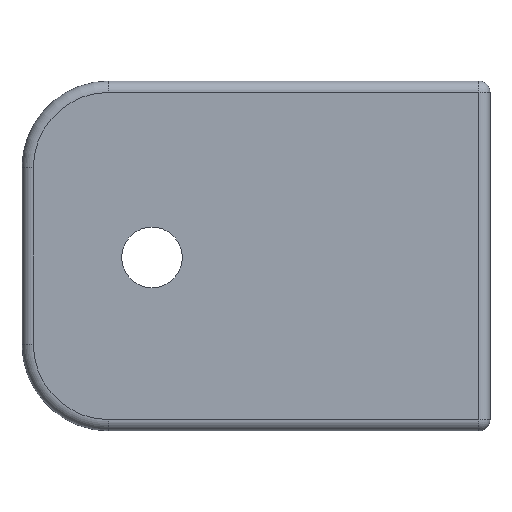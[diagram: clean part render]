
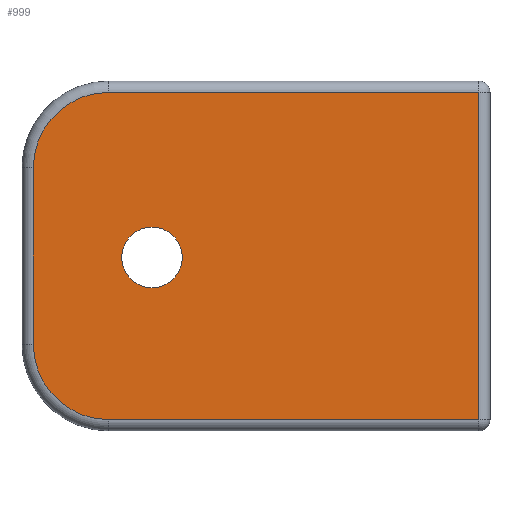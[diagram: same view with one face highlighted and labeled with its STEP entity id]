
A CAD part, front view. The second image highlights one B-rep face of the part: STEP entity #999.
In plain terms, the highlighted planar face has unit normal (0, -1, 0).
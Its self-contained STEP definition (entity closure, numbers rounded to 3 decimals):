
#17=FACE_BOUND('',#346,.T.);
#29=PLANE('',#1100);
#57=LINE('',#1514,#152);
#85=LINE('',#1604,#180);
#86=LINE('',#1608,#181);
#87=LINE('',#1612,#182);
#152=VECTOR('',#1199,10.);
#180=VECTOR('',#1291,10.);
#181=VECTOR('',#1296,10.);
#182=VECTOR('',#1299,10.);
#286=FACE_OUTER_BOUND('',#345,.T.);
#345=EDGE_LOOP('',(#765,#766,#767,#768,#769,#770));
#346=EDGE_LOOP('',(#771));
#413=CIRCLE('',#1101,6.62);
#414=CIRCLE('',#1102,6.62);
#415=CIRCLE('',#1103,2.667);
#442=VERTEX_POINT('',#1511);
#443=VERTEX_POINT('',#1513);
#473=VERTEX_POINT('',#1603);
#474=VERTEX_POINT('',#1607);
#475=VERTEX_POINT('',#1609);
#476=VERTEX_POINT('',#1611);
#477=VERTEX_POINT('',#1614);
#538=EDGE_CURVE('',#442,#443,#57,.T.);
#583=EDGE_CURVE('',#443,#473,#85,.T.);
#585=EDGE_CURVE('',#474,#442,#86,.T.);
#586=EDGE_CURVE('',#475,#474,#413,.T.);
#587=EDGE_CURVE('',#476,#475,#87,.T.);
#588=EDGE_CURVE('',#473,#476,#414,.T.);
#589=EDGE_CURVE('',#477,#477,#415,.T.);
#765=ORIENTED_EDGE('',*,*,#538,.F.);
#766=ORIENTED_EDGE('',*,*,#585,.F.);
#767=ORIENTED_EDGE('',*,*,#586,.F.);
#768=ORIENTED_EDGE('',*,*,#587,.F.);
#769=ORIENTED_EDGE('',*,*,#588,.F.);
#770=ORIENTED_EDGE('',*,*,#583,.F.);
#771=ORIENTED_EDGE('',*,*,#589,.T.);
#999=ADVANCED_FACE('',(#286,#17),#29,.F.);
#1100=AXIS2_PLACEMENT_3D('',#1606,#1294,#1295);
#1101=AXIS2_PLACEMENT_3D('',#1610,#1297,#1298);
#1102=AXIS2_PLACEMENT_3D('',#1613,#1300,#1301);
#1103=AXIS2_PLACEMENT_3D('',#1615,#1302,#1303);
#1199=DIRECTION('',(0.,0.,-1.));
#1291=DIRECTION('',(-1.,0.,0.));
#1294=DIRECTION('center_axis',(0.,1.,0.));
#1295=DIRECTION('ref_axis',(0.,0.,1.));
#1296=DIRECTION('',(1.,0.,0.));
#1297=DIRECTION('center_axis',(0.,1.,0.));
#1298=DIRECTION('ref_axis',(-0.707,0.,0.707));
#1299=DIRECTION('',(0.,0.,1.));
#1300=DIRECTION('center_axis',(0.,1.,0.));
#1301=DIRECTION('ref_axis',(-0.707,0.,-0.707));
#1302=DIRECTION('center_axis',(0.,1.,0.));
#1303=DIRECTION('ref_axis',(-1.,0.,0.));
#1511=CARTESIAN_POINT('',(40.01,-0.25,0.));
#1513=CARTESIAN_POINT('',(40.01,-0.25,-28.778));
#1514=CARTESIAN_POINT('',(40.01,-0.25,-7.195));
#1603=CARTESIAN_POINT('',(7.46,-0.25,-28.778));
#1604=CARTESIAN_POINT('',(29.489,-0.25,-28.778));
#1606=CARTESIAN_POINT('Origin',(19.66,-0.25,-14.389));
#1607=CARTESIAN_POINT('',(7.46,-0.25,0.));
#1608=CARTESIAN_POINT('',(9.83,-0.25,0.));
#1609=CARTESIAN_POINT('',(0.84,-0.25,-6.62));
#1610=CARTESIAN_POINT('Origin',(7.46,-0.25,-6.62));
#1611=CARTESIAN_POINT('',(0.84,-0.25,-22.158));
#1612=CARTESIAN_POINT('',(0.84,-0.25,-21.584));
#1613=CARTESIAN_POINT('Origin',(7.46,-0.25,-22.158));
#1614=CARTESIAN_POINT('',(13.944,-0.25,-14.516));
#1615=CARTESIAN_POINT('Origin',(11.277,-0.25,-14.516));
